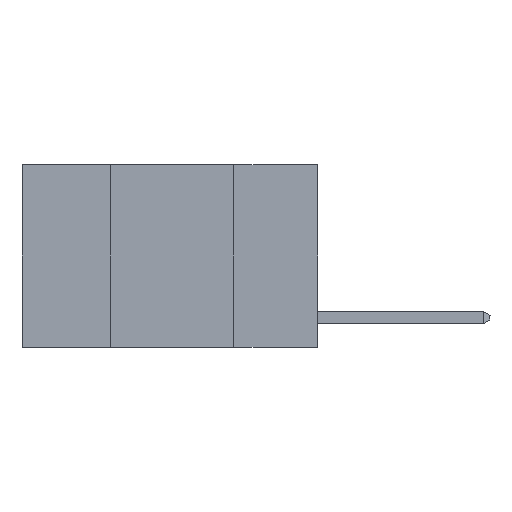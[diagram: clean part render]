
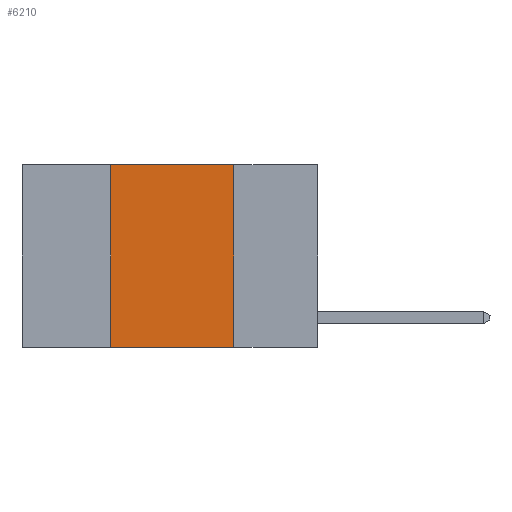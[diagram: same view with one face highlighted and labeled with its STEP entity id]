
A CAD part, left-side view. The second image highlights one B-rep face of the part: STEP entity #6210.
In plain terms, the highlighted planar face has unit normal (-1, 0, 0).
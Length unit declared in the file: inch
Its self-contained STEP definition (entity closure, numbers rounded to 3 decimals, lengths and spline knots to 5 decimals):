
#98 = ORIENTED_EDGE ( 'NONE', *, *, #26679, .F. ) ;
#3196 = VERTEX_POINT ( 'NONE', #23162 ) ;
#3643 = DIRECTION ( 'NONE',  ( 0., 0., -1. ) ) ;
#4078 = CARTESIAN_POINT ( 'NONE',  ( 0., 0.42, 0. ) ) ;
#4287 = DIRECTION ( 'NONE',  ( 0., -1., 0. ) ) ;
#4827 = ORIENTED_EDGE ( 'NONE', *, *, #21902, .T. ) ;
#5274 = LINE ( 'NONE', #18386, #14151 ) ;
#5343 = CARTESIAN_POINT ( 'NONE',  ( 0., 0.42, -0.37 ) ) ;
#6051 = VECTOR ( 'NONE', #4287, 39.37008 ) ;
#6210 = ADVANCED_FACE ( 'NONE', ( #8345 ), #21033, .F. ) ;
#6849 = CARTESIAN_POINT ( 'NONE',  ( 0., 0.6, -0.37 ) ) ;
#8064 = DIRECTION ( 'NONE',  ( 1., 0., 0. ) ) ;
#8092 = DIRECTION ( 'NONE',  ( 0., -1., 0. ) ) ;
#8153 = CARTESIAN_POINT ( 'NONE',  ( 0., 0.17, -0.37 ) ) ;
#8345 = FACE_OUTER_BOUND ( 'NONE', #13564, .T. ) ;
#10527 = CARTESIAN_POINT ( 'NONE',  ( 0., 0.6, 0. ) ) ;
#11968 = VECTOR ( 'NONE', #8092, 39.37008 ) ;
#13471 = ORIENTED_EDGE ( 'NONE', *, *, #20271, .F. ) ;
#13564 = EDGE_LOOP ( 'NONE', ( #18505, #13471, #98, #4827 ) ) ;
#13970 = DIRECTION ( 'NONE',  ( 0., 0., 1. ) ) ;
#14151 = VECTOR ( 'NONE', #13970, 39.37008 ) ;
#14399 = DIRECTION ( 'NONE',  ( 0., 0., -1. ) ) ;
#15140 = VERTEX_POINT ( 'NONE', #8153 ) ;
#16524 = CARTESIAN_POINT ( 'NONE',  ( 0., 0.17, 0. ) ) ;
#17038 = CARTESIAN_POINT ( 'NONE',  ( 0., 0.6, 0. ) ) ;
#17391 = VECTOR ( 'NONE', #14399, 39.37008 ) ;
#17683 = LINE ( 'NONE', #6849, #6051 ) ;
#18386 = CARTESIAN_POINT ( 'NONE',  ( 0., 0.42, 0. ) ) ;
#18505 = ORIENTED_EDGE ( 'NONE', *, *, #28011, .F. ) ;
#18643 = AXIS2_PLACEMENT_3D ( 'NONE', #17038, #8064, #3643 ) ;
#20271 = EDGE_CURVE ( 'NONE', #23800, #3196, #21203, .T. ) ;
#21033 = PLANE ( 'NONE',  #18643 ) ;
#21203 = LINE ( 'NONE', #10527, #11968 ) ;
#21902 = EDGE_CURVE ( 'NONE', #26869, #15140, #17683, .T. ) ;
#23162 = CARTESIAN_POINT ( 'NONE',  ( 0., 0.17, 0. ) ) ;
#23800 = VERTEX_POINT ( 'NONE', #4078 ) ;
#26679 = EDGE_CURVE ( 'NONE', #26869, #23800, #5274, .T. ) ;
#26869 = VERTEX_POINT ( 'NONE', #5343 ) ;
#27322 = LINE ( 'NONE', #16524, #17391 ) ;
#28011 = EDGE_CURVE ( 'NONE', #3196, #15140, #27322, .T. ) ;
